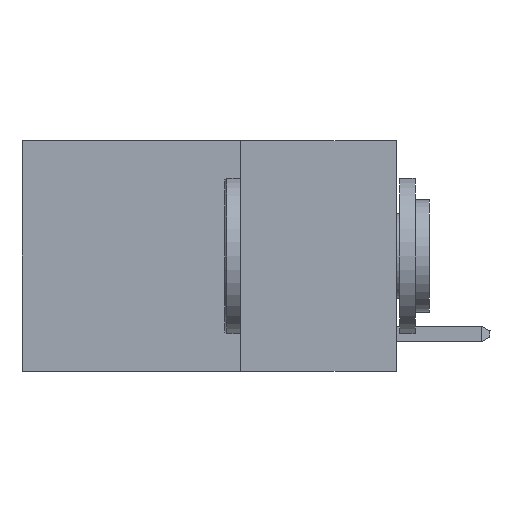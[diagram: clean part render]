
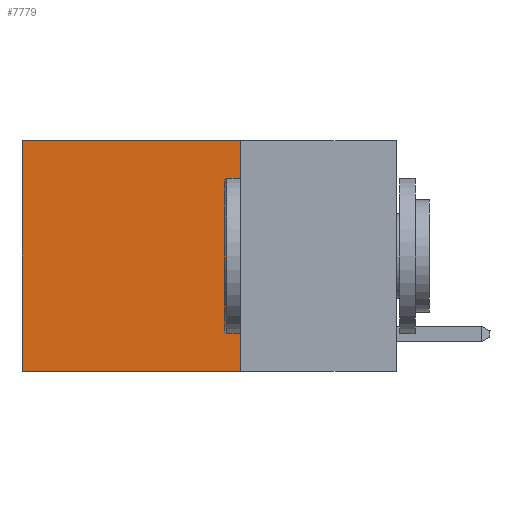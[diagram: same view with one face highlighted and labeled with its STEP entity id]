
A CAD part, left-side view. The second image highlights one B-rep face of the part: STEP entity #7779.
In plain terms, the highlighted planar face has unit normal (-1, 0, 0).
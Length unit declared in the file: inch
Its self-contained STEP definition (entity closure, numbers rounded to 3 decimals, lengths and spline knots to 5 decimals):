
#130 = DIRECTION ( 'NONE',  ( 1., 0., 0. ) ) ;
#273 = VECTOR ( 'NONE', #16889, 39.37008 ) ;
#1410 = PLANE ( 'NONE',  #1561 ) ;
#1525 = CARTESIAN_POINT ( 'NONE',  ( 0.2625, 0.25, 0. ) ) ;
#1561 = AXIS2_PLACEMENT_3D ( 'NONE', #11865, #130, #4167 ) ;
#2868 = FACE_OUTER_BOUND ( 'NONE', #12936, .T. ) ;
#4163 = CARTESIAN_POINT ( 'NONE',  ( 0.2625, 0.6, -0.37 ) ) ;
#4167 = DIRECTION ( 'NONE',  ( 0., 0., -1. ) ) ;
#4262 = DIRECTION ( 'NONE',  ( 0., 1., 0. ) ) ;
#4704 = DIRECTION ( 'NONE',  ( 0., 0., -1. ) ) ;
#6452 = VERTEX_POINT ( 'NONE', #4163 ) ;
#6526 = VERTEX_POINT ( 'NONE', #10497 ) ;
#6590 = VERTEX_POINT ( 'NONE', #13155 ) ;
#7309 = VECTOR ( 'NONE', #12068, 39.37008 ) ;
#7779 = ADVANCED_FACE ( 'NONE', ( #2868 ), #1410, .F. ) ;
#7809 = LINE ( 'NONE', #1525, #7309 ) ;
#8999 = EDGE_CURVE ( 'NONE', #6590, #16328, #10746, .T. ) ;
#9836 = CARTESIAN_POINT ( 'NONE',  ( 0.2625, 0.6, 0. ) ) ;
#10268 = CARTESIAN_POINT ( 'NONE',  ( 0.2625, 0.6, 0. ) ) ;
#10497 = CARTESIAN_POINT ( 'NONE',  ( 0.2625, 0.25, -0.37 ) ) ;
#10746 = LINE ( 'NONE', #15991, #273 ) ;
#10835 = CARTESIAN_POINT ( 'NONE',  ( 0.2625, 0.25, -0.37 ) ) ;
#11306 = VECTOR ( 'NONE', #4704, 39.37008 ) ;
#11865 = CARTESIAN_POINT ( 'NONE',  ( 0.2625, 0.25, 0. ) ) ;
#12068 = DIRECTION ( 'NONE',  ( 0., 0., -1. ) ) ;
#12409 = EDGE_CURVE ( 'NONE', #6590, #6526, #7809, .T. ) ;
#12765 = ORIENTED_EDGE ( 'NONE', *, *, #8999, .T. ) ;
#12936 = EDGE_LOOP ( 'NONE', ( #16606, #14683, #13468, #12765 ) ) ;
#12962 = EDGE_CURVE ( 'NONE', #6526, #6452, #13743, .T. ) ;
#13155 = CARTESIAN_POINT ( 'NONE',  ( 0.2625, 0.25, 0. ) ) ;
#13468 = ORIENTED_EDGE ( 'NONE', *, *, #12409, .F. ) ;
#13607 = LINE ( 'NONE', #9836, #11306 ) ;
#13743 = LINE ( 'NONE', #10835, #14655 ) ;
#14655 = VECTOR ( 'NONE', #4262, 39.37008 ) ;
#14683 = ORIENTED_EDGE ( 'NONE', *, *, #12962, .F. ) ;
#15991 = CARTESIAN_POINT ( 'NONE',  ( 0.2625, 0.25, 0. ) ) ;
#16114 = EDGE_CURVE ( 'NONE', #16328, #6452, #13607, .T. ) ;
#16328 = VERTEX_POINT ( 'NONE', #10268 ) ;
#16606 = ORIENTED_EDGE ( 'NONE', *, *, #16114, .T. ) ;
#16889 = DIRECTION ( 'NONE',  ( 0., 1., 0. ) ) ;
